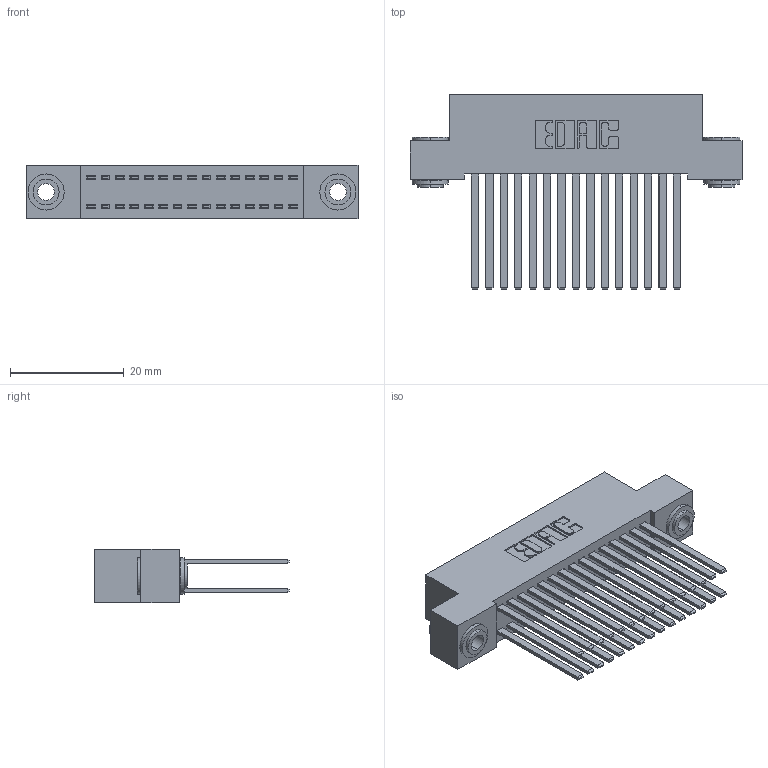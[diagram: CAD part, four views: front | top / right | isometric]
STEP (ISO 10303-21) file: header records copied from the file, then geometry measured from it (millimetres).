
FILE_DESCRIPTION (( 'STEP AP203' ), '1' );
FILE_NAME ('342-030-544-203.STEP', '2018-08-11T15:43:42', ( '' ), ( '' ), 'SwSTEP 2.0', 'SolidWorks 2016', '' );
FILE_SCHEMA (( 'CONFIG_CONTROL_DESIGN' ));
Length unit declared in the file: inch
Products named in the file (4): 342-030-544-203; 342 Part_.156 TH; 345-292-001_345-293-144; 342-250-002_345-250-002-102
Assembly tree (33 placements, depth 2):
  342-030-544-203
    342 Part_.156 TH
    345-292-001_345-293-144  x30
    342-250-002_345-250-002-102  x2
Bounding box: 58.42 x 34.3 x 9.4 mm (x, y, z)
Volume: 5564.6 mm3; surface area: 9771.2 mm2
Topology: 33 solids, 33 shells, 1528 faces, 4485 edges, 2946 vertices
Faces by surface type: plane 1036, cylinder 484, cone 8
Entity records: 13476 total; most frequent: CARTESIAN_POINT 2237, ORIENTED_EDGE 2166, DIRECTION 1989, EDGE_CURVE 1083, VECTOR 935, LINE 935, VERTEX_POINT 718, AXIS2_PLACEMENT_3D 527
